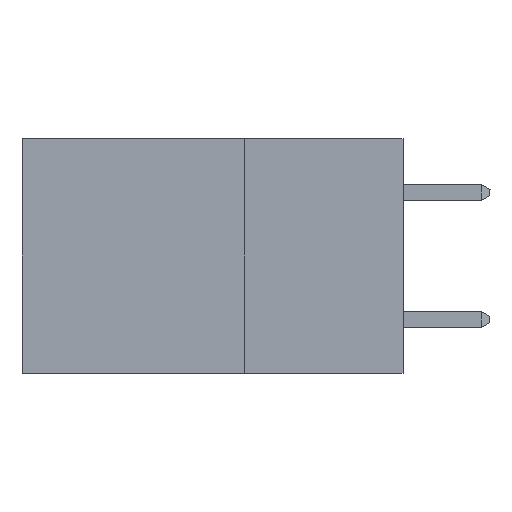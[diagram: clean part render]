
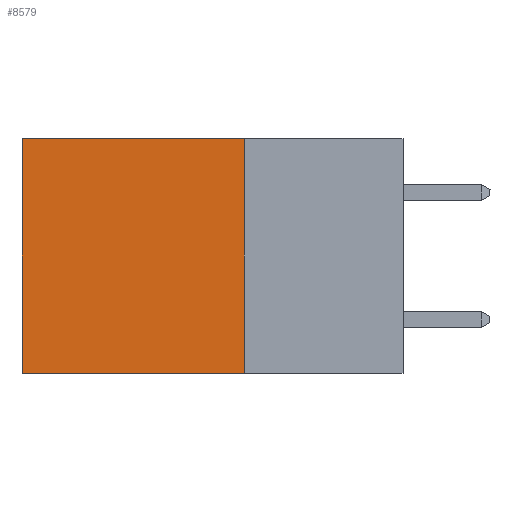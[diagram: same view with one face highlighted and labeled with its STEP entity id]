
A CAD part, left-side view. The second image highlights one B-rep face of the part: STEP entity #8579.
In plain terms, the highlighted planar face has unit normal (-1, 0, 0).
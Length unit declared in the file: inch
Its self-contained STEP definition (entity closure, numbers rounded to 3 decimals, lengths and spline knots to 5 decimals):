
#248 = VECTOR ( 'NONE', #13873, 39.37008 ) ;
#1238 = VERTEX_POINT ( 'NONE', #16997 ) ;
#1391 = EDGE_CURVE ( 'NONE', #11170, #1238, #9079, .T. ) ;
#1617 = CARTESIAN_POINT ( 'NONE',  ( 0.2875, 0.25, 0. ) ) ;
#2002 = DIRECTION ( 'NONE',  ( 0., 0., -1. ) ) ;
#2305 = VECTOR ( 'NONE', #2002, 39.37008 ) ;
#2826 = LINE ( 'NONE', #8540, #2305 ) ;
#3257 = DIRECTION ( 'NONE',  ( 0., 0., -1. ) ) ;
#4309 = VECTOR ( 'NONE', #19605, 39.37008 ) ;
#4708 = AXIS2_PLACEMENT_3D ( 'NONE', #1617, #13228, #3257 ) ;
#5063 = VERTEX_POINT ( 'NONE', #19654 ) ;
#7165 = DIRECTION ( 'NONE',  ( 0., 0., -1. ) ) ;
#7685 = CARTESIAN_POINT ( 'NONE',  ( 0.2875, 0.25, 0. ) ) ;
#8540 = CARTESIAN_POINT ( 'NONE',  ( 0.2875, 0.6, 0. ) ) ;
#8579 = ADVANCED_FACE ( 'NONE', ( #18015 ), #19730, .F. ) ;
#8880 = CARTESIAN_POINT ( 'NONE',  ( 0.2875, 0.25, 0. ) ) ;
#9079 = LINE ( 'NONE', #14564, #248 ) ;
#9299 = LINE ( 'NONE', #7685, #4309 ) ;
#9636 = VERTEX_POINT ( 'NONE', #12406 ) ;
#10396 = ORIENTED_EDGE ( 'NONE', *, *, #16304, .T. ) ;
#10871 = EDGE_CURVE ( 'NONE', #9636, #11170, #17196, .T. ) ;
#11170 = VERTEX_POINT ( 'NONE', #11541 ) ;
#11541 = CARTESIAN_POINT ( 'NONE',  ( 0.2875, 0.25, -0.37 ) ) ;
#12406 = CARTESIAN_POINT ( 'NONE',  ( 0.2875, 0.25, 0. ) ) ;
#13228 = DIRECTION ( 'NONE',  ( 1., 0., 0. ) ) ;
#13541 = ORIENTED_EDGE ( 'NONE', *, *, #1391, .F. ) ;
#13873 = DIRECTION ( 'NONE',  ( 0., 1., 0. ) ) ;
#14564 = CARTESIAN_POINT ( 'NONE',  ( 0.2875, 0.25, -0.37 ) ) ;
#16304 = EDGE_CURVE ( 'NONE', #5063, #1238, #2826, .T. ) ;
#16937 = ORIENTED_EDGE ( 'NONE', *, *, #10871, .F. ) ;
#16997 = CARTESIAN_POINT ( 'NONE',  ( 0.2875, 0.6, -0.37 ) ) ;
#17196 = LINE ( 'NONE', #8880, #20430 ) ;
#17453 = EDGE_CURVE ( 'NONE', #9636, #5063, #9299, .T. ) ;
#18015 = FACE_OUTER_BOUND ( 'NONE', #21223, .T. ) ;
#18441 = ORIENTED_EDGE ( 'NONE', *, *, #17453, .T. ) ;
#19605 = DIRECTION ( 'NONE',  ( 0., 1., 0. ) ) ;
#19654 = CARTESIAN_POINT ( 'NONE',  ( 0.2875, 0.6, 0. ) ) ;
#19730 = PLANE ( 'NONE',  #4708 ) ;
#20430 = VECTOR ( 'NONE', #7165, 39.37008 ) ;
#21223 = EDGE_LOOP ( 'NONE', ( #10396, #13541, #16937, #18441 ) ) ;
